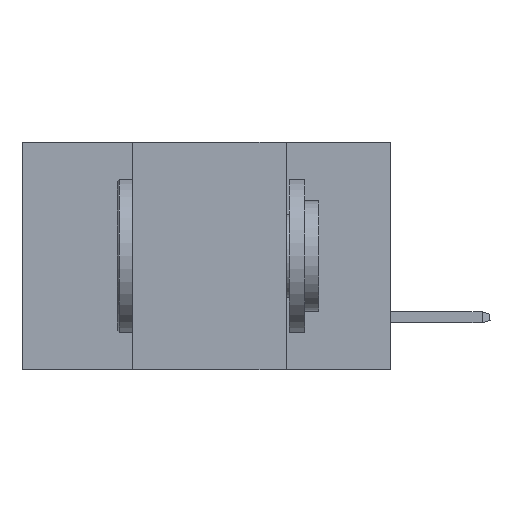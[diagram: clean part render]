
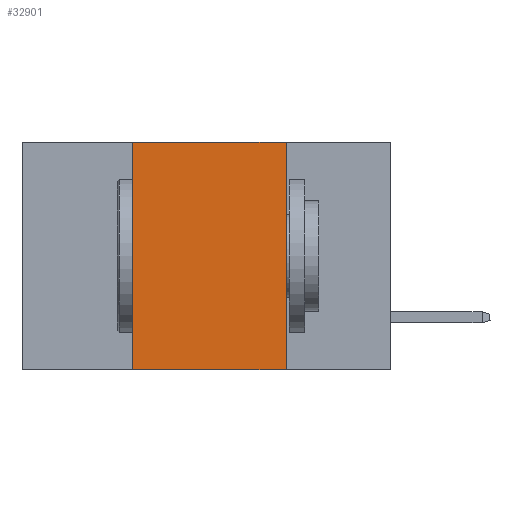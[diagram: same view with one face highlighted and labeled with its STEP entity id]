
A CAD part, left-side view. The second image highlights one B-rep face of the part: STEP entity #32901.
In plain terms, the highlighted planar face has unit normal (-1, 0, 0).
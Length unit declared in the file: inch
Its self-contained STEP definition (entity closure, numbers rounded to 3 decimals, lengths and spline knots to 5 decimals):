
#117 = LINE ( 'NONE', #26519, #21584 ) ;
#433 = DIRECTION ( 'NONE',  ( 1., 0., 0. ) ) ;
#1045 = EDGE_CURVE ( 'NONE', #33389, #36761, #2384, .T. ) ;
#1490 = ORIENTED_EDGE ( 'NONE', *, *, #32781, .T. ) ;
#2016 = CARTESIAN_POINT ( 'NONE',  ( 0., 0.42, 0. ) ) ;
#2384 = LINE ( 'NONE', #2016, #16176 ) ;
#2900 = DIRECTION ( 'NONE',  ( 0., -1., 0. ) ) ;
#3630 = CARTESIAN_POINT ( 'NONE',  ( 0., 0.17, -0.37 ) ) ;
#4359 = VERTEX_POINT ( 'NONE', #16981 ) ;
#4875 = DIRECTION ( 'NONE',  ( 0., 0., -1. ) ) ;
#5175 = DIRECTION ( 'NONE',  ( 0., 0., 1. ) ) ;
#6218 = EDGE_LOOP ( 'NONE', ( #41868, #30559, #32161, #1490 ) ) ;
#8790 = LINE ( 'NONE', #13767, #39941 ) ;
#13165 = EDGE_CURVE ( 'NONE', #4359, #32157, #8790, .T. ) ;
#13578 = CARTESIAN_POINT ( 'NONE',  ( 0., 0.6, 0. ) ) ;
#13767 = CARTESIAN_POINT ( 'NONE',  ( 0., 0.17, 0. ) ) ;
#14394 = FACE_OUTER_BOUND ( 'NONE', #6218, .T. ) ;
#16176 = VECTOR ( 'NONE', #5175, 39.37008 ) ;
#16417 = DIRECTION ( 'NONE',  ( 0., 0., -1. ) ) ;
#16750 = CARTESIAN_POINT ( 'NONE',  ( 0., 0.42, -0.37 ) ) ;
#16981 = CARTESIAN_POINT ( 'NONE',  ( 0., 0.17, 0. ) ) ;
#17742 = CARTESIAN_POINT ( 'NONE',  ( 0., 0.42, 0. ) ) ;
#20040 = DIRECTION ( 'NONE',  ( 0., -1., 0. ) ) ;
#21584 = VECTOR ( 'NONE', #20040, 39.37008 ) ;
#22429 = CARTESIAN_POINT ( 'NONE',  ( 0., 0.6, -0.37 ) ) ;
#25697 = VECTOR ( 'NONE', #2900, 39.37008 ) ;
#26519 = CARTESIAN_POINT ( 'NONE',  ( 0., 0.6, 0. ) ) ;
#30559 = ORIENTED_EDGE ( 'NONE', *, *, #32353, .F. ) ;
#32157 = VERTEX_POINT ( 'NONE', #3630 ) ;
#32161 = ORIENTED_EDGE ( 'NONE', *, *, #1045, .F. ) ;
#32353 = EDGE_CURVE ( 'NONE', #36761, #4359, #117, .T. ) ;
#32718 = PLANE ( 'NONE',  #40001 ) ;
#32781 = EDGE_CURVE ( 'NONE', #33389, #32157, #34334, .T. ) ;
#32901 = ADVANCED_FACE ( 'NONE', ( #14394 ), #32718, .F. ) ;
#33389 = VERTEX_POINT ( 'NONE', #16750 ) ;
#34334 = LINE ( 'NONE', #22429, #25697 ) ;
#36761 = VERTEX_POINT ( 'NONE', #17742 ) ;
#39941 = VECTOR ( 'NONE', #4875, 39.37008 ) ;
#40001 = AXIS2_PLACEMENT_3D ( 'NONE', #13578, #433, #16417 ) ;
#41868 = ORIENTED_EDGE ( 'NONE', *, *, #13165, .F. ) ;
